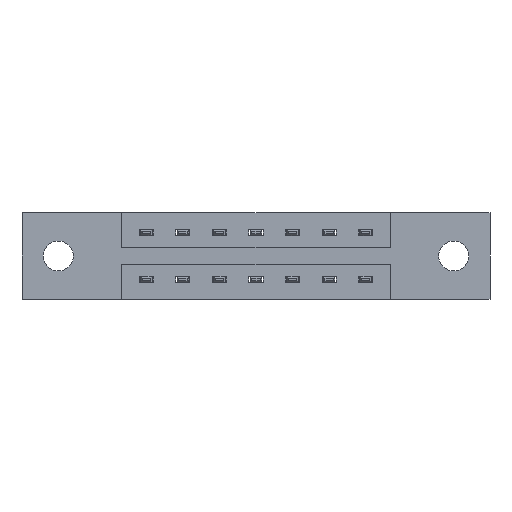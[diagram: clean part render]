
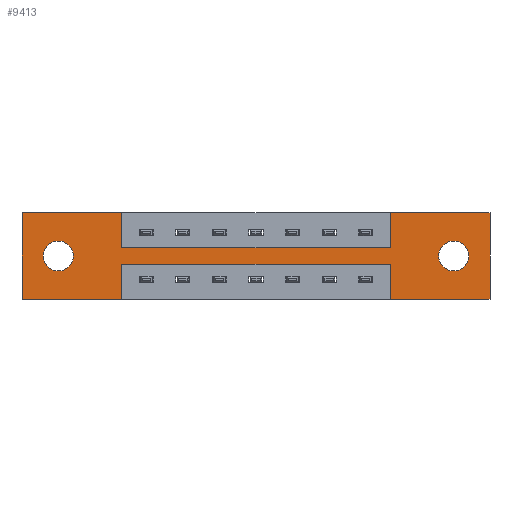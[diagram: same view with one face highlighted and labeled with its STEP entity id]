
A CAD part, front view. The second image highlights one B-rep face of the part: STEP entity #9413.
In plain terms, the highlighted planar face has unit normal (0, -1, 0).
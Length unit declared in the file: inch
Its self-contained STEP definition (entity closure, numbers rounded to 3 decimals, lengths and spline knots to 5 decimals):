
#8 = ORIENTED_EDGE ( 'NONE', *, *, #785, .F. ) ;
#100 = CARTESIAN_POINT ( 'NONE',  ( 0., 0., 0. ) ) ;
#147 = EDGE_CURVE ( 'NONE', #751, #6778, #7275, .T. ) ;
#153 = CARTESIAN_POINT ( 'NONE',  ( 0.425, 0., -0.37 ) ) ;
#204 = ORIENTED_EDGE ( 'NONE', *, *, #5846, .T. ) ;
#365 = VERTEX_POINT ( 'NONE', #4025 ) ;
#482 = VECTOR ( 'NONE', #3567, 39.37008 ) ;
#503 = ORIENTED_EDGE ( 'NONE', *, *, #3558, .F. ) ;
#514 = AXIS2_PLACEMENT_3D ( 'NONE', #1125, #6435, #2647 ) ;
#527 = CARTESIAN_POINT ( 'NONE',  ( 1.573, 0., 0. ) ) ;
#563 = EDGE_CURVE ( 'NONE', #6354, #6241, #2760, .T. ) ;
#583 = DIRECTION ( 'NONE',  ( 0., 0., 1. ) ) ;
#635 = EDGE_LOOP ( 'NONE', ( #3507, #204 ) ) ;
#661 = CARTESIAN_POINT ( 'NONE',  ( 0., 0., 0. ) ) ;
#751 = VERTEX_POINT ( 'NONE', #527 ) ;
#774 = AXIS2_PLACEMENT_3D ( 'NONE', #2758, #1920, #2041 ) ;
#785 = EDGE_CURVE ( 'NONE', #8702, #9102, #2265, .T. ) ;
#926 = CARTESIAN_POINT ( 'NONE',  ( 0.155, 0., -0.249 ) ) ;
#1060 = EDGE_CURVE ( 'NONE', #1061, #6199, #1915, .T. ) ;
#1061 = VERTEX_POINT ( 'NONE', #2126 ) ;
#1125 = CARTESIAN_POINT ( 'NONE',  ( 0.155, 0., -0.185 ) ) ;
#1176 = LINE ( 'NONE', #6193, #7930 ) ;
#1330 = EDGE_CURVE ( 'NONE', #2797, #8597, #4767, .T. ) ;
#1358 = CARTESIAN_POINT ( 'NONE',  ( 1.573, 0., -0.37 ) ) ;
#1506 = DIRECTION ( 'NONE',  ( 0., -1., 0. ) ) ;
#1603 = VECTOR ( 'NONE', #2084, 39.37008 ) ;
#1876 = LINE ( 'NONE', #8390, #6136 ) ;
#1915 = CIRCLE ( 'NONE', #514, 0.064 ) ;
#1920 = DIRECTION ( 'NONE',  ( 0., 1., 0. ) ) ;
#2041 = DIRECTION ( 'NONE',  ( 0., 0., -1. ) ) ;
#2084 = DIRECTION ( 'NONE',  ( 0., 0., 1. ) ) ;
#2126 = CARTESIAN_POINT ( 'NONE',  ( 0.155, 0., -0.121 ) ) ;
#2177 = VERTEX_POINT ( 'NONE', #4330 ) ;
#2196 = CARTESIAN_POINT ( 'NONE',  ( 1.843, 0., -0.121 ) ) ;
#2265 = LINE ( 'NONE', #8887, #9562 ) ;
#2372 = DIRECTION ( 'NONE',  ( 0., 0., -1. ) ) ;
#2452 = CARTESIAN_POINT ( 'NONE',  ( 0.425, 0., -0.22 ) ) ;
#2532 = CARTESIAN_POINT ( 'NONE',  ( 0., 0., -0.37 ) ) ;
#2622 = DIRECTION ( 'NONE',  ( -1., 0., 0. ) ) ;
#2642 = ORIENTED_EDGE ( 'NONE', *, *, #3698, .T. ) ;
#2647 = DIRECTION ( 'NONE',  ( 0., 0., 1. ) ) ;
#2758 = CARTESIAN_POINT ( 'NONE',  ( 1.843, 0., -0.185 ) ) ;
#2760 = CIRCLE ( 'NONE', #7609, 0.064 ) ;
#2797 = VERTEX_POINT ( 'NONE', #661 ) ;
#2997 = VERTEX_POINT ( 'NONE', #153 ) ;
#3051 = VECTOR ( 'NONE', #4503, 39.37008 ) ;
#3128 = CARTESIAN_POINT ( 'NONE',  ( 0.425, 0., 0. ) ) ;
#3160 = EDGE_CURVE ( 'NONE', #2177, #8883, #8835, .T. ) ;
#3507 = ORIENTED_EDGE ( 'NONE', *, *, #1060, .T. ) ;
#3558 = EDGE_CURVE ( 'NONE', #2997, #365, #5901, .T. ) ;
#3567 = DIRECTION ( 'NONE',  ( 1., 0., 0. ) ) ;
#3698 = EDGE_CURVE ( 'NONE', #6241, #6354, #7921, .T. ) ;
#3853 = EDGE_CURVE ( 'NONE', #8597, #2177, #1876, .T. ) ;
#3974 = CIRCLE ( 'NONE', #8564, 0.064 ) ;
#4025 = CARTESIAN_POINT ( 'NONE',  ( 0., 0., -0.37 ) ) ;
#4098 = FACE_BOUND ( 'NONE', #635, .T. ) ;
#4131 = AXIS2_PLACEMENT_3D ( 'NONE', #4523, #1506, #9782 ) ;
#4200 = ORIENTED_EDGE ( 'NONE', *, *, #8430, .F. ) ;
#4327 = ORIENTED_EDGE ( 'NONE', *, *, #563, .T. ) ;
#4330 = CARTESIAN_POINT ( 'NONE',  ( 0.425, 0., -0.15 ) ) ;
#4503 = DIRECTION ( 'NONE',  ( 0., 0., -1. ) ) ;
#4523 = CARTESIAN_POINT ( 'NONE',  ( 0., 0., -0.37 ) ) ;
#4567 = EDGE_CURVE ( 'NONE', #6778, #8702, #6604, .T. ) ;
#4575 = ORIENTED_EDGE ( 'NONE', *, *, #147, .F. ) ;
#4690 = CARTESIAN_POINT ( 'NONE',  ( 0.425, 0., -0.22 ) ) ;
#4767 = LINE ( 'NONE', #5780, #482 ) ;
#4824 = CARTESIAN_POINT ( 'NONE',  ( 1.998, 0., -0.37 ) ) ;
#5020 = VECTOR ( 'NONE', #6176, 39.37008 ) ;
#5054 = LINE ( 'NONE', #6733, #5393 ) ;
#5143 = ORIENTED_EDGE ( 'NONE', *, *, #3853, .F. ) ;
#5312 = PLANE ( 'NONE',  #4131 ) ;
#5393 = VECTOR ( 'NONE', #583, 39.37008 ) ;
#5558 = CARTESIAN_POINT ( 'NONE',  ( 0.155, 0., -0.185 ) ) ;
#5697 = EDGE_LOOP ( 'NONE', ( #9246, #6819, #8081, #8, #7099, #4575, #9768, #9247, #5143, #9539, #4200, #503 ) ) ;
#5780 = CARTESIAN_POINT ( 'NONE',  ( 0., 0., 0. ) ) ;
#5846 = EDGE_CURVE ( 'NONE', #6199, #1061, #3974, .T. ) ;
#5901 = LINE ( 'NONE', #2532, #7452 ) ;
#5927 = CARTESIAN_POINT ( 'NONE',  ( 1.998, 0., 0. ) ) ;
#6136 = VECTOR ( 'NONE', #2372, 39.37008 ) ;
#6176 = DIRECTION ( 'NONE',  ( 1., 0., 0. ) ) ;
#6193 = CARTESIAN_POINT ( 'NONE',  ( 1.573, 0., 0. ) ) ;
#6199 = VERTEX_POINT ( 'NONE', #926 ) ;
#6201 = EDGE_CURVE ( 'NONE', #8883, #751, #1176, .T. ) ;
#6233 = DIRECTION ( 'NONE',  ( 0., 0., 1. ) ) ;
#6239 = EDGE_CURVE ( 'NONE', #8690, #9605, #6519, .T. ) ;
#6241 = VERTEX_POINT ( 'NONE', #6987 ) ;
#6299 = CARTESIAN_POINT ( 'NONE',  ( 1.843, 0., -0.185 ) ) ;
#6354 = VERTEX_POINT ( 'NONE', #2196 ) ;
#6374 = DIRECTION ( 'NONE',  ( 0., 0., -1. ) ) ;
#6435 = DIRECTION ( 'NONE',  ( 0., 1., 0. ) ) ;
#6519 = LINE ( 'NONE', #2452, #6737 ) ;
#6604 = LINE ( 'NONE', #7892, #8453 ) ;
#6733 = CARTESIAN_POINT ( 'NONE',  ( 0., 0., 0. ) ) ;
#6737 = VECTOR ( 'NONE', #7751, 39.37008 ) ;
#6778 = VERTEX_POINT ( 'NONE', #5927 ) ;
#6819 = ORIENTED_EDGE ( 'NONE', *, *, #6239, .F. ) ;
#6854 = VECTOR ( 'NONE', #9350, 39.37008 ) ;
#6987 = CARTESIAN_POINT ( 'NONE',  ( 1.843, 0., -0.249 ) ) ;
#7090 = CARTESIAN_POINT ( 'NONE',  ( 0.425, 0., -0.15 ) ) ;
#7099 = ORIENTED_EDGE ( 'NONE', *, *, #4567, .F. ) ;
#7275 = LINE ( 'NONE', #100, #5020 ) ;
#7365 = CARTESIAN_POINT ( 'NONE',  ( 1.573, 0., -0.37 ) ) ;
#7434 = LINE ( 'NONE', #8244, #3051 ) ;
#7452 = VECTOR ( 'NONE', #2622, 39.37008 ) ;
#7553 = LINE ( 'NONE', #1358, #1603 ) ;
#7596 = EDGE_CURVE ( 'NONE', #9605, #2997, #7434, .T. ) ;
#7609 = AXIS2_PLACEMENT_3D ( 'NONE', #6299, #8578, #6374 ) ;
#7703 = DIRECTION ( 'NONE',  ( 0., 0., 1. ) ) ;
#7751 = DIRECTION ( 'NONE',  ( -1., 0., 0. ) ) ;
#7754 = FACE_BOUND ( 'NONE', #9116, .T. ) ;
#7878 = FACE_OUTER_BOUND ( 'NONE', #5697, .T. ) ;
#7892 = CARTESIAN_POINT ( 'NONE',  ( 1.998, 0., 0. ) ) ;
#7921 = CIRCLE ( 'NONE', #774, 0.064 ) ;
#7930 = VECTOR ( 'NONE', #6233, 39.37008 ) ;
#8069 = CARTESIAN_POINT ( 'NONE',  ( 1.573, 0., -0.15 ) ) ;
#8081 = ORIENTED_EDGE ( 'NONE', *, *, #8484, .F. ) ;
#8244 = CARTESIAN_POINT ( 'NONE',  ( 0.425, 0., -0.37 ) ) ;
#8390 = CARTESIAN_POINT ( 'NONE',  ( 0.425, 0., 0. ) ) ;
#8430 = EDGE_CURVE ( 'NONE', #365, #2797, #5054, .T. ) ;
#8453 = VECTOR ( 'NONE', #9296, 39.37008 ) ;
#8484 = EDGE_CURVE ( 'NONE', #9102, #8690, #7553, .T. ) ;
#8493 = DIRECTION ( 'NONE',  ( 0., 1., 0. ) ) ;
#8564 = AXIS2_PLACEMENT_3D ( 'NONE', #5558, #8493, #7703 ) ;
#8578 = DIRECTION ( 'NONE',  ( 0., 1., 0. ) ) ;
#8597 = VERTEX_POINT ( 'NONE', #3128 ) ;
#8690 = VERTEX_POINT ( 'NONE', #9232 ) ;
#8702 = VERTEX_POINT ( 'NONE', #4824 ) ;
#8835 = LINE ( 'NONE', #7090, #6854 ) ;
#8883 = VERTEX_POINT ( 'NONE', #8069 ) ;
#8887 = CARTESIAN_POINT ( 'NONE',  ( 0., 0., -0.37 ) ) ;
#9102 = VERTEX_POINT ( 'NONE', #7365 ) ;
#9116 = EDGE_LOOP ( 'NONE', ( #4327, #2642 ) ) ;
#9232 = CARTESIAN_POINT ( 'NONE',  ( 1.573, 0., -0.22 ) ) ;
#9246 = ORIENTED_EDGE ( 'NONE', *, *, #7596, .F. ) ;
#9247 = ORIENTED_EDGE ( 'NONE', *, *, #3160, .F. ) ;
#9296 = DIRECTION ( 'NONE',  ( 0., 0., -1. ) ) ;
#9350 = DIRECTION ( 'NONE',  ( 1., 0., 0. ) ) ;
#9413 = ADVANCED_FACE ( 'NONE', ( #7754, #4098, #7878 ), #5312, .T. ) ;
#9539 = ORIENTED_EDGE ( 'NONE', *, *, #1330, .F. ) ;
#9562 = VECTOR ( 'NONE', #9654, 39.37008 ) ;
#9605 = VERTEX_POINT ( 'NONE', #4690 ) ;
#9654 = DIRECTION ( 'NONE',  ( -1., 0., 0. ) ) ;
#9768 = ORIENTED_EDGE ( 'NONE', *, *, #6201, .F. ) ;
#9782 = DIRECTION ( 'NONE',  ( 0., 0., -1. ) ) ;
